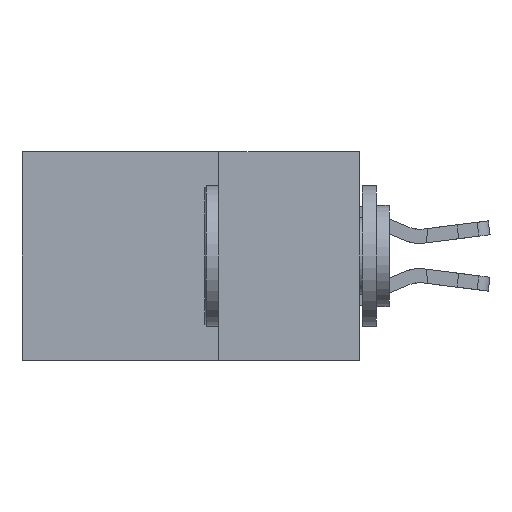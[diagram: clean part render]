
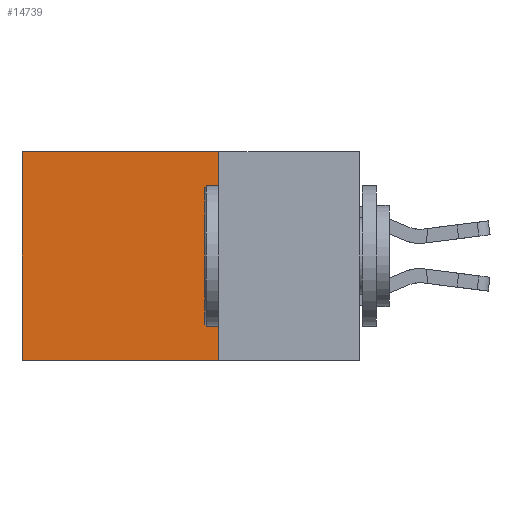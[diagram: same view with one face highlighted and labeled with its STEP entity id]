
A CAD part, left-side view. The second image highlights one B-rep face of the part: STEP entity #14739.
In plain terms, the highlighted planar face has unit normal (-1, 0, 0).
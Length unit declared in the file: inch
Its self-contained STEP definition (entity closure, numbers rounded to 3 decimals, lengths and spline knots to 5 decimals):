
#365 = CARTESIAN_POINT ( 'NONE',  ( 0.2875, 0.25, 0. ) ) ;
#413 = FACE_OUTER_BOUND ( 'NONE', #17666, .T. ) ;
#1413 = ORIENTED_EDGE ( 'NONE', *, *, #15703, .T. ) ;
#1942 = DIRECTION ( 'NONE',  ( 0., 1., 0. ) ) ;
#2198 = PLANE ( 'NONE',  #22033 ) ;
#2494 = EDGE_CURVE ( 'NONE', #15671, #7741, #20369, .T. ) ;
#2902 = DIRECTION ( 'NONE',  ( 0., 0., -1. ) ) ;
#5183 = EDGE_CURVE ( 'NONE', #15671, #17902, #19457, .T. ) ;
#5525 = CARTESIAN_POINT ( 'NONE',  ( 0.2875, 0.25, -0.37 ) ) ;
#5696 = DIRECTION ( 'NONE',  ( 1., 0., 0. ) ) ;
#6205 = VECTOR ( 'NONE', #1942, 39.37008 ) ;
#7741 = VERTEX_POINT ( 'NONE', #14050 ) ;
#7866 = DIRECTION ( 'NONE',  ( 0., 1., 0. ) ) ;
#8070 = LINE ( 'NONE', #8271, #12247 ) ;
#8271 = CARTESIAN_POINT ( 'NONE',  ( 0.2875, 0.6, 0. ) ) ;
#8321 = VECTOR ( 'NONE', #20058, 39.37008 ) ;
#8552 = ORIENTED_EDGE ( 'NONE', *, *, #9326, .F. ) ;
#9326 = EDGE_CURVE ( 'NONE', #17902, #18380, #10112, .T. ) ;
#9377 = ORIENTED_EDGE ( 'NONE', *, *, #5183, .F. ) ;
#10112 = LINE ( 'NONE', #18520, #18980 ) ;
#12247 = VECTOR ( 'NONE', #2902, 39.37008 ) ;
#14050 = CARTESIAN_POINT ( 'NONE',  ( 0.2875, 0.6, 0. ) ) ;
#14739 = ADVANCED_FACE ( 'NONE', ( #413 ), #2198, .F. ) ;
#15671 = VERTEX_POINT ( 'NONE', #18839 ) ;
#15703 = EDGE_CURVE ( 'NONE', #7741, #18380, #8070, .T. ) ;
#16294 = CARTESIAN_POINT ( 'NONE',  ( 0.2875, 0.25, 0. ) ) ;
#17666 = EDGE_LOOP ( 'NONE', ( #1413, #8552, #9377, #20190 ) ) ;
#17902 = VERTEX_POINT ( 'NONE', #5525 ) ;
#18084 = DIRECTION ( 'NONE',  ( 0., 0., -1. ) ) ;
#18255 = CARTESIAN_POINT ( 'NONE',  ( 0.2875, 0.25, 0. ) ) ;
#18380 = VERTEX_POINT ( 'NONE', #22597 ) ;
#18520 = CARTESIAN_POINT ( 'NONE',  ( 0.2875, 0.25, -0.37 ) ) ;
#18839 = CARTESIAN_POINT ( 'NONE',  ( 0.2875, 0.25, 0. ) ) ;
#18980 = VECTOR ( 'NONE', #7866, 39.37008 ) ;
#19457 = LINE ( 'NONE', #18255, #8321 ) ;
#20058 = DIRECTION ( 'NONE',  ( 0., 0., -1. ) ) ;
#20190 = ORIENTED_EDGE ( 'NONE', *, *, #2494, .T. ) ;
#20369 = LINE ( 'NONE', #365, #6205 ) ;
#22033 = AXIS2_PLACEMENT_3D ( 'NONE', #16294, #5696, #18084 ) ;
#22597 = CARTESIAN_POINT ( 'NONE',  ( 0.2875, 0.6, -0.37 ) ) ;
